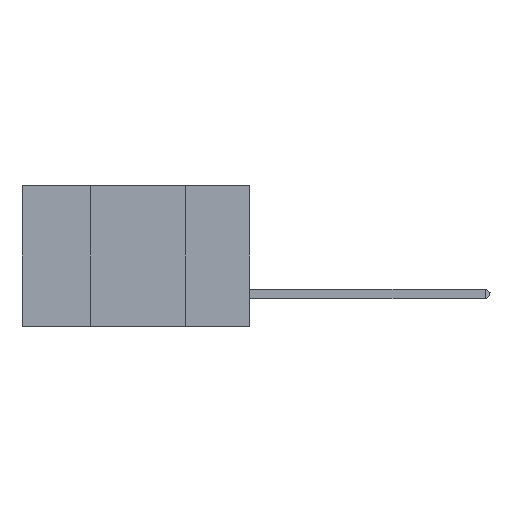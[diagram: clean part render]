
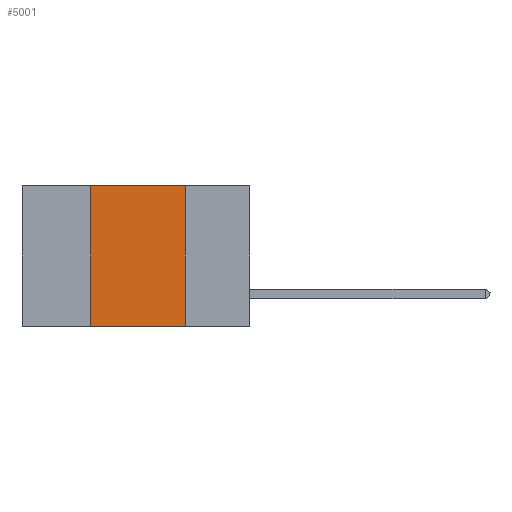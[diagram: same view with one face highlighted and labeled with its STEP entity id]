
A CAD part, left-side view. The second image highlights one B-rep face of the part: STEP entity #5001.
In plain terms, the highlighted planar face has unit normal (-1, 0, 0).
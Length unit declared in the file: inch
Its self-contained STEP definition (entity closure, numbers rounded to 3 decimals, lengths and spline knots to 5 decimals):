
#52 = EDGE_LOOP ( 'NONE', ( #23042, #27878, #22400, #15132 ) ) ;
#423 = CARTESIAN_POINT ( 'NONE',  ( 0., 0.42, 0. ) ) ;
#821 = PLANE ( 'NONE',  #23108 ) ;
#2722 = EDGE_CURVE ( 'NONE', #14648, #28795, #16128, .T. ) ;
#3135 = DIRECTION ( 'NONE',  ( 0., 0., -1. ) ) ;
#5001 = ADVANCED_FACE ( 'NONE', ( #11233 ), #821, .F. ) ;
#5217 = CARTESIAN_POINT ( 'NONE',  ( 0., 0.17, 0. ) ) ;
#5926 = EDGE_CURVE ( 'NONE', #28795, #27835, #11531, .T. ) ;
#5975 = EDGE_CURVE ( 'NONE', #17135, #14648, #24747, .T. ) ;
#5987 = CARTESIAN_POINT ( 'NONE',  ( 0., 0.42, 0. ) ) ;
#9463 = VECTOR ( 'NONE', #18422, 39.37008 ) ;
#10433 = VECTOR ( 'NONE', #18615, 39.37008 ) ;
#11233 = FACE_OUTER_BOUND ( 'NONE', #52, .T. ) ;
#11531 = LINE ( 'NONE', #27216, #11884 ) ;
#11755 = DIRECTION ( 'NONE',  ( 0., -1., 0. ) ) ;
#11884 = VECTOR ( 'NONE', #27318, 39.37008 ) ;
#14648 = VERTEX_POINT ( 'NONE', #423 ) ;
#15132 = ORIENTED_EDGE ( 'NONE', *, *, #25734, .T. ) ;
#16128 = LINE ( 'NONE', #22924, #9463 ) ;
#17135 = VERTEX_POINT ( 'NONE', #21503 ) ;
#17271 = DIRECTION ( 'NONE',  ( 1., 0., 0. ) ) ;
#18422 = DIRECTION ( 'NONE',  ( 0., -1., 0. ) ) ;
#18615 = DIRECTION ( 'NONE',  ( 0., 0., 1. ) ) ;
#20848 = VECTOR ( 'NONE', #11755, 39.37008 ) ;
#21503 = CARTESIAN_POINT ( 'NONE',  ( 0., 0.42, -0.37 ) ) ;
#21728 = CARTESIAN_POINT ( 'NONE',  ( 0., 0.6, 0. ) ) ;
#22400 = ORIENTED_EDGE ( 'NONE', *, *, #5975, .F. ) ;
#22924 = CARTESIAN_POINT ( 'NONE',  ( 0., 0.6, 0. ) ) ;
#23042 = ORIENTED_EDGE ( 'NONE', *, *, #5926, .F. ) ;
#23108 = AXIS2_PLACEMENT_3D ( 'NONE', #21728, #17271, #3135 ) ;
#24747 = LINE ( 'NONE', #5987, #10433 ) ;
#25734 = EDGE_CURVE ( 'NONE', #17135, #27835, #29374, .T. ) ;
#25809 = CARTESIAN_POINT ( 'NONE',  ( 0., 0.6, -0.37 ) ) ;
#26940 = CARTESIAN_POINT ( 'NONE',  ( 0., 0.17, -0.37 ) ) ;
#27216 = CARTESIAN_POINT ( 'NONE',  ( 0., 0.17, 0. ) ) ;
#27318 = DIRECTION ( 'NONE',  ( 0., 0., -1. ) ) ;
#27835 = VERTEX_POINT ( 'NONE', #26940 ) ;
#27878 = ORIENTED_EDGE ( 'NONE', *, *, #2722, .F. ) ;
#28795 = VERTEX_POINT ( 'NONE', #5217 ) ;
#29374 = LINE ( 'NONE', #25809, #20848 ) ;
